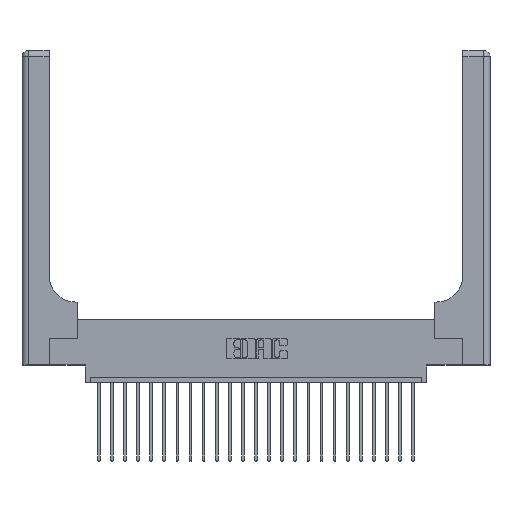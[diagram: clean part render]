
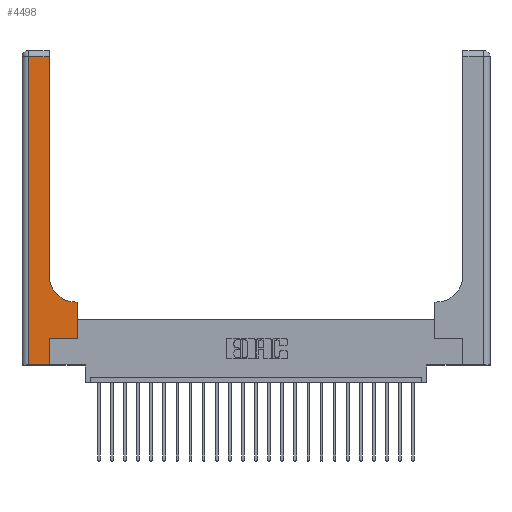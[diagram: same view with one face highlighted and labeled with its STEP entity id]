
A CAD part, top view. The second image highlights one B-rep face of the part: STEP entity #4498.
In plain terms, the highlighted planar face has unit normal (0, 0, 1).
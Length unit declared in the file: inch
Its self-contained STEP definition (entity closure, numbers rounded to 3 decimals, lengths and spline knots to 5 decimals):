
#9 = LINE ( 'NONE', #14567, #8531 ) ;
#779 = CARTESIAN_POINT ( 'NONE',  ( 0.265, 0., 0.37 ) ) ;
#946 = LINE ( 'NONE', #13945, #21063 ) ;
#1018 = VECTOR ( 'NONE', #7436, 39.37008 ) ;
#1574 = DIRECTION ( 'NONE',  ( -1., 0., 0. ) ) ;
#1691 = FACE_OUTER_BOUND ( 'NONE', #11229, .T. ) ;
#2492 = CARTESIAN_POINT ( 'NONE',  ( 0.26, 2.94, 0.37 ) ) ;
#2710 = EDGE_CURVE ( 'NONE', #22776, #19440, #12934, .T. ) ;
#2997 = CARTESIAN_POINT ( 'NONE',  ( 0.26, 0.85, 0.37 ) ) ;
#3852 = LINE ( 'NONE', #5644, #1018 ) ;
#4246 = DIRECTION ( 'NONE',  ( 0., 1., 0. ) ) ;
#4498 = ADVANCED_FACE ( 'NONE', ( #1691 ), #10413, .F. ) ;
#4563 = CARTESIAN_POINT ( 'NONE',  ( 0.06, 0., 0.37 ) ) ;
#4610 = EDGE_CURVE ( 'NONE', #16158, #9066, #9, .T. ) ;
#4852 = VECTOR ( 'NONE', #1574, 39.37008 ) ;
#5011 = CARTESIAN_POINT ( 'NONE',  ( 0.06, 2.94, 0.37 ) ) ;
#5228 = VECTOR ( 'NONE', #7142, 39.37008 ) ;
#5353 = LINE ( 'NONE', #21579, #5228 ) ;
#5644 = CARTESIAN_POINT ( 'NONE',  ( 0., 0., 0.37 ) ) ;
#6230 = EDGE_CURVE ( 'NONE', #23349, #18953, #946, .T. ) ;
#6667 = CARTESIAN_POINT ( 'NONE',  ( 0.51, 0.85, 0.37 ) ) ;
#6725 = ORIENTED_EDGE ( 'NONE', *, *, #14848, .T. ) ;
#7142 = DIRECTION ( 'NONE',  ( 0., 1., 0. ) ) ;
#7436 = DIRECTION ( 'NONE',  ( 1., 0., 0. ) ) ;
#8391 = LINE ( 'NONE', #15654, #4852 ) ;
#8491 = ORIENTED_EDGE ( 'NONE', *, *, #20653, .T. ) ;
#8531 = VECTOR ( 'NONE', #16702, 39.37008 ) ;
#9066 = VERTEX_POINT ( 'NONE', #20397 ) ;
#9748 = LINE ( 'NONE', #779, #19112 ) ;
#10413 = PLANE ( 'NONE',  #16132 ) ;
#10503 = DIRECTION ( 'NONE',  ( 0., 1., 0. ) ) ;
#10731 = CARTESIAN_POINT ( 'NONE',  ( 0.26, 3., 0.37 ) ) ;
#10746 = CARTESIAN_POINT ( 'NONE',  ( 0.265, 0., 0.37 ) ) ;
#10757 = DIRECTION ( 'NONE',  ( -1., 0., 0. ) ) ;
#11229 = EDGE_LOOP ( 'NONE', ( #22339, #21622, #15113, #6725, #8491, #14615, #11754, #21736, #12294 ) ) ;
#11300 = VERTEX_POINT ( 'NONE', #2997 ) ;
#11754 = ORIENTED_EDGE ( 'NONE', *, *, #13921, .T. ) ;
#11805 = DIRECTION ( 'NONE',  ( 1., 0., 0. ) ) ;
#11852 = CARTESIAN_POINT ( 'NONE',  ( 0.528, 0.6, 0.37 ) ) ;
#11989 = CARTESIAN_POINT ( 'NONE',  ( 0.528, 0.25, 0.37 ) ) ;
#12294 = ORIENTED_EDGE ( 'NONE', *, *, #21982, .T. ) ;
#12608 = CARTESIAN_POINT ( 'NONE',  ( 0.265, 0.25, 0.37 ) ) ;
#12934 = LINE ( 'NONE', #20214, #15790 ) ;
#13447 = VERTEX_POINT ( 'NONE', #2492 ) ;
#13921 = EDGE_CURVE ( 'NONE', #18953, #16158, #5353, .T. ) ;
#13945 = CARTESIAN_POINT ( 'NONE',  ( 0.265, 0.25, 0.37 ) ) ;
#13963 = LINE ( 'NONE', #10731, #16403 ) ;
#14044 = DIRECTION ( 'NONE',  ( 0., 0., -1. ) ) ;
#14490 = AXIS2_PLACEMENT_3D ( 'NONE', #6667, #14044, #15716 ) ;
#14567 = CARTESIAN_POINT ( 'NONE',  ( 0.26, 0.6, 0.37 ) ) ;
#14615 = ORIENTED_EDGE ( 'NONE', *, *, #6230, .T. ) ;
#14848 = EDGE_CURVE ( 'NONE', #19440, #18446, #3852, .T. ) ;
#15113 = ORIENTED_EDGE ( 'NONE', *, *, #2710, .T. ) ;
#15261 = EDGE_CURVE ( 'NONE', #13447, #22776, #8391, .T. ) ;
#15654 = CARTESIAN_POINT ( 'NONE',  ( 0., 2.94, 0.37 ) ) ;
#15716 = DIRECTION ( 'NONE',  ( 1., 0., 0. ) ) ;
#15777 = DIRECTION ( 'NONE',  ( 0., 0., -1. ) ) ;
#15790 = VECTOR ( 'NONE', #16399, 39.37008 ) ;
#16132 = AXIS2_PLACEMENT_3D ( 'NONE', #23511, #15777, #10757 ) ;
#16158 = VERTEX_POINT ( 'NONE', #11852 ) ;
#16399 = DIRECTION ( 'NONE',  ( 0., -1., 0. ) ) ;
#16403 = VECTOR ( 'NONE', #10503, 39.37008 ) ;
#16702 = DIRECTION ( 'NONE',  ( -1., 0., 0. ) ) ;
#18446 = VERTEX_POINT ( 'NONE', #10746 ) ;
#18953 = VERTEX_POINT ( 'NONE', #11989 ) ;
#19112 = VECTOR ( 'NONE', #4246, 39.37008 ) ;
#19440 = VERTEX_POINT ( 'NONE', #4563 ) ;
#20214 = CARTESIAN_POINT ( 'NONE',  ( 0.06, 3., 0.37 ) ) ;
#20397 = CARTESIAN_POINT ( 'NONE',  ( 0.51, 0.6, 0.37 ) ) ;
#20653 = EDGE_CURVE ( 'NONE', #18446, #23349, #9748, .T. ) ;
#20960 = CIRCLE ( 'NONE', #14490, 0.25 ) ;
#21063 = VECTOR ( 'NONE', #11805, 39.37008 ) ;
#21579 = CARTESIAN_POINT ( 'NONE',  ( 0.528, 0.25, 0.37 ) ) ;
#21622 = ORIENTED_EDGE ( 'NONE', *, *, #15261, .T. ) ;
#21736 = ORIENTED_EDGE ( 'NONE', *, *, #4610, .T. ) ;
#21982 = EDGE_CURVE ( 'NONE', #9066, #11300, #20960, .T. ) ;
#22339 = ORIENTED_EDGE ( 'NONE', *, *, #22828, .T. ) ;
#22776 = VERTEX_POINT ( 'NONE', #5011 ) ;
#22828 = EDGE_CURVE ( 'NONE', #11300, #13447, #13963, .T. ) ;
#23349 = VERTEX_POINT ( 'NONE', #12608 ) ;
#23511 = CARTESIAN_POINT ( 'NONE',  ( 0., 3., 0.37 ) ) ;
